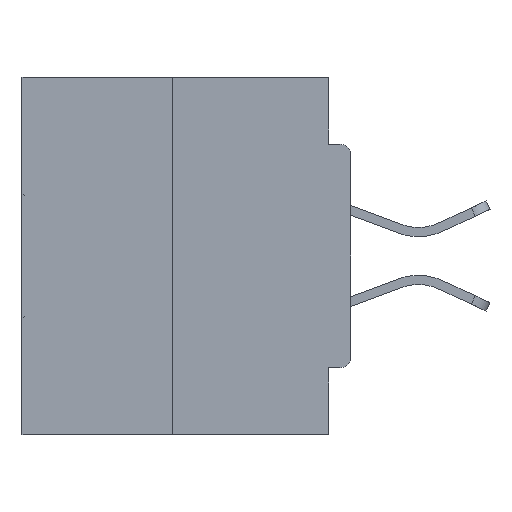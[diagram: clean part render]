
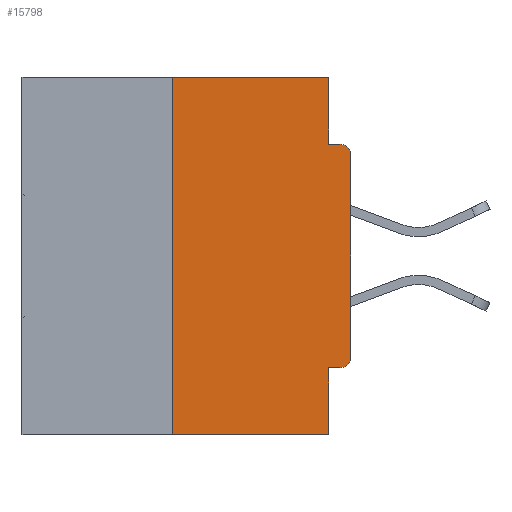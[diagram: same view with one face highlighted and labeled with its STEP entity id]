
A CAD part, left-side view. The second image highlights one B-rep face of the part: STEP entity #15798.
In plain terms, the highlighted planar face has unit normal (-1, 0, 0).
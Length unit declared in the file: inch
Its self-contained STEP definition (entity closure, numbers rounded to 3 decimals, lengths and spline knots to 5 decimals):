
#189 = PLANE ( 'NONE',  #36845 ) ;
#331 = EDGE_CURVE ( 'NONE', #16323, #36850, #741, .T. ) ;
#553 = CARTESIAN_POINT ( 'NONE',  ( 0., 0.46, 0. ) ) ;
#741 = CIRCLE ( 'NONE', #26477, 0.015 ) ;
#1795 = DIRECTION ( 'NONE',  ( 0., 0., -1. ) ) ;
#2829 = ORIENTED_EDGE ( 'NONE', *, *, #24002, .T. ) ;
#2908 = AXIS2_PLACEMENT_3D ( 'NONE', #30726, #40027, #1795 ) ;
#2938 = ORIENTED_EDGE ( 'NONE', *, *, #40542, .F. ) ;
#3068 = DIRECTION ( 'NONE',  ( 0., 0., -1. ) ) ;
#3877 = LINE ( 'NONE', #35780, #30406 ) ;
#4792 = CARTESIAN_POINT ( 'NONE',  ( 0., 0.031, -0.5 ) ) ;
#5388 = VECTOR ( 'NONE', #13725, 39.37008 ) ;
#6173 = ORIENTED_EDGE ( 'NONE', *, *, #19577, .F. ) ;
#6703 = DIRECTION ( 'NONE',  ( 0., -1., 0. ) ) ;
#6848 = EDGE_CURVE ( 'NONE', #38625, #15135, #36541, .T. ) ;
#7081 = VECTOR ( 'NONE', #40668, 39.37008 ) ;
#7886 = LINE ( 'NONE', #33758, #18849 ) ;
#7979 = CARTESIAN_POINT ( 'NONE',  ( 0., 0., 0. ) ) ;
#9802 = ORIENTED_EDGE ( 'NONE', *, *, #6848, .F. ) ;
#9875 = VERTEX_POINT ( 'NONE', #35242 ) ;
#9938 = DIRECTION ( 'NONE',  ( 0., 0., -1. ) ) ;
#11108 = VERTEX_POINT ( 'NONE', #26624 ) ;
#11703 = DIRECTION ( 'NONE',  ( 0., -1., 0. ) ) ;
#12196 = CARTESIAN_POINT ( 'NONE',  ( 0., 0., -0.3915 ) ) ;
#12323 = LINE ( 'NONE', #553, #29353 ) ;
#12608 = VERTEX_POINT ( 'NONE', #36367 ) ;
#13725 = DIRECTION ( 'NONE',  ( 0., 0., 1. ) ) ;
#14020 = VECTOR ( 'NONE', #27421, 39.37008 ) ;
#14290 = CARTESIAN_POINT ( 'NONE',  ( 0., 0.031, -0.5 ) ) ;
#15117 = CARTESIAN_POINT ( 'NONE',  ( 0., 0.031, 0. ) ) ;
#15135 = VERTEX_POINT ( 'NONE', #4792 ) ;
#15634 = CARTESIAN_POINT ( 'NONE',  ( 0., 0.25, 0. ) ) ;
#15637 = ORIENTED_EDGE ( 'NONE', *, *, #26512, .F. ) ;
#15798 = ADVANCED_FACE ( 'NONE', ( #34208 ), #189, .F. ) ;
#16323 = VERTEX_POINT ( 'NONE', #16839 ) ;
#16839 = CARTESIAN_POINT ( 'NONE',  ( 0., 0.015, -0.4065 ) ) ;
#17017 = ORIENTED_EDGE ( 'NONE', *, *, #22550, .F. ) ;
#18026 = VERTEX_POINT ( 'NONE', #15634 ) ;
#18849 = VECTOR ( 'NONE', #11703, 39.37008 ) ;
#18964 = DIRECTION ( 'NONE',  ( -1., 0., 0. ) ) ;
#19577 = EDGE_CURVE ( 'NONE', #12608, #27850, #23091, .T. ) ;
#21077 = CARTESIAN_POINT ( 'NONE',  ( 0., 0.46, -0.5 ) ) ;
#21758 = CARTESIAN_POINT ( 'NONE',  ( 0., 0.015, -0.3915 ) ) ;
#22550 = EDGE_CURVE ( 'NONE', #11108, #18026, #24387, .T. ) ;
#23091 = LINE ( 'NONE', #15117, #7081 ) ;
#24002 = EDGE_CURVE ( 'NONE', #36850, #30463, #24028, .T. ) ;
#24028 = LINE ( 'NONE', #7979, #14020 ) ;
#24237 = DIRECTION ( 'NONE',  ( 0., 0., -1. ) ) ;
#24301 = DIRECTION ( 'NONE',  ( 0., -1., 0. ) ) ;
#24387 = LINE ( 'NONE', #36485, #5388 ) ;
#25252 = ORIENTED_EDGE ( 'NONE', *, *, #40522, .T. ) ;
#26477 = AXIS2_PLACEMENT_3D ( 'NONE', #21758, #18964, #3068 ) ;
#26512 = EDGE_CURVE ( 'NONE', #18026, #12608, #12323, .T. ) ;
#26624 = CARTESIAN_POINT ( 'NONE',  ( 0., 0.25, -0.5 ) ) ;
#26925 = VECTOR ( 'NONE', #24301, 39.37008 ) ;
#27421 = DIRECTION ( 'NONE',  ( 0., 0., 1. ) ) ;
#27850 = VERTEX_POINT ( 'NONE', #36549 ) ;
#27928 = EDGE_CURVE ( 'NONE', #30463, #9875, #35173, .T. ) ;
#28290 = CARTESIAN_POINT ( 'NONE',  ( 0., 0., -0.1085 ) ) ;
#29092 = DIRECTION ( 'NONE',  ( 1., 0., 0. ) ) ;
#29213 = ORIENTED_EDGE ( 'NONE', *, *, #331, .T. ) ;
#29353 = VECTOR ( 'NONE', #6703, 39.37008 ) ;
#29722 = CARTESIAN_POINT ( 'NONE',  ( 0., 0.031, -0.4065 ) ) ;
#30406 = VECTOR ( 'NONE', #38453, 39.37008 ) ;
#30463 = VERTEX_POINT ( 'NONE', #28290 ) ;
#30635 = EDGE_CURVE ( 'NONE', #16323, #38625, #3877, .T. ) ;
#30726 = CARTESIAN_POINT ( 'NONE',  ( 0., 0.015, -0.1085 ) ) ;
#32017 = CARTESIAN_POINT ( 'NONE',  ( 0., 0.46, 0. ) ) ;
#33758 = CARTESIAN_POINT ( 'NONE',  ( 0., 0., -0.0935 ) ) ;
#34208 = FACE_OUTER_BOUND ( 'NONE', #39825, .T. ) ;
#35173 = CIRCLE ( 'NONE', #2908, 0.015 ) ;
#35242 = CARTESIAN_POINT ( 'NONE',  ( 0., 0.015, -0.0935 ) ) ;
#35351 = LINE ( 'NONE', #21077, #26925 ) ;
#35763 = ORIENTED_EDGE ( 'NONE', *, *, #30635, .F. ) ;
#35780 = CARTESIAN_POINT ( 'NONE',  ( 0., 0., -0.4065 ) ) ;
#36367 = CARTESIAN_POINT ( 'NONE',  ( 0., 0.031, 0. ) ) ;
#36485 = CARTESIAN_POINT ( 'NONE',  ( 0., 0.25, 0. ) ) ;
#36541 = LINE ( 'NONE', #14290, #37551 ) ;
#36549 = CARTESIAN_POINT ( 'NONE',  ( 0., 0.031, -0.0935 ) ) ;
#36845 = AXIS2_PLACEMENT_3D ( 'NONE', #32017, #29092, #9938 ) ;
#36850 = VERTEX_POINT ( 'NONE', #12196 ) ;
#37551 = VECTOR ( 'NONE', #24237, 39.37008 ) ;
#38453 = DIRECTION ( 'NONE',  ( 0., 1., 0. ) ) ;
#38625 = VERTEX_POINT ( 'NONE', #29722 ) ;
#39825 = EDGE_LOOP ( 'NONE', ( #15637, #17017, #25252, #9802, #35763, #29213, #2829, #40614, #2938, #6173 ) ) ;
#40027 = DIRECTION ( 'NONE',  ( -1., 0., 0. ) ) ;
#40522 = EDGE_CURVE ( 'NONE', #11108, #15135, #35351, .T. ) ;
#40542 = EDGE_CURVE ( 'NONE', #27850, #9875, #7886, .T. ) ;
#40614 = ORIENTED_EDGE ( 'NONE', *, *, #27928, .T. ) ;
#40668 = DIRECTION ( 'NONE',  ( 0., 0., -1. ) ) ;
